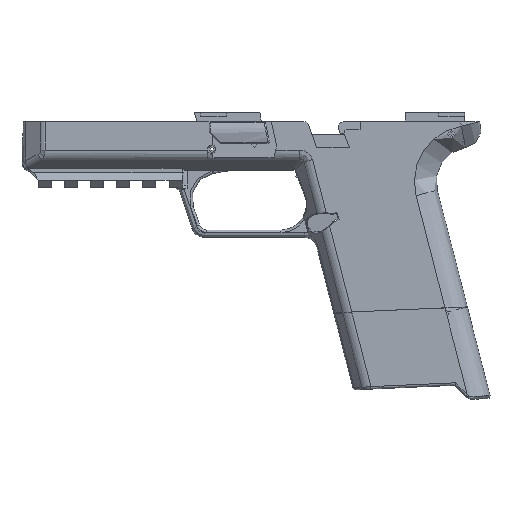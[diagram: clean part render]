
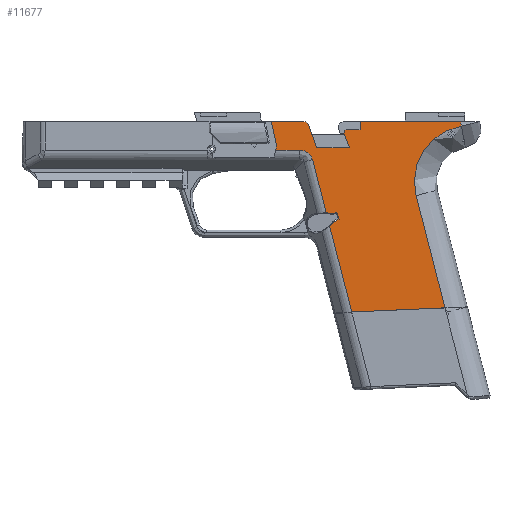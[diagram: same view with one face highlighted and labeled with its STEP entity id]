
A CAD part, left-side view. The second image highlights one B-rep face of the part: STEP entity #11677.
In plain terms, the highlighted face is planar.
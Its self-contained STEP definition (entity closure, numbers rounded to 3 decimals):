
#155=ELLIPSE('',#12633,10.693,7.);
#763=PLANE('',#12628);
#1239=FACE_OUTER_BOUND('',#1904,.T.);
#1904=EDGE_LOOP('',(#9328,#9329,#9330,#9331,#9332,#9333,#9334,#9335,#9336,
#9337,#9338,#9339,#9340,#9341,#9342,#9343,#9344,#9345,#9346,#9347,#9348,
#9349,#9350,#9351,#9352));
#2806=LINE('',#19325,#3937);
#2812=LINE('',#19335,#3943);
#2816=LINE('',#19343,#3947);
#2827=LINE('',#19402,#3958);
#2853=LINE('',#19467,#3984);
#2854=LINE('',#19469,#3985);
#2855=LINE('',#19471,#3986);
#2856=LINE('',#19477,#3987);
#2857=LINE('',#19479,#3988);
#2858=LINE('',#19481,#3989);
#2859=LINE('',#19485,#3990);
#2860=LINE('',#19487,#3991);
#2861=LINE('',#19489,#3992);
#2862=LINE('',#19493,#3993);
#2863=LINE('',#19495,#3994);
#2864=LINE('',#19497,#3995);
#2865=LINE('',#19499,#3996);
#2866=LINE('',#19502,#3997);
#3937=VECTOR('',#14691,10.);
#3943=VECTOR('',#14701,10.);
#3947=VECTOR('',#14709,10.);
#3958=VECTOR('',#14742,10.);
#3984=VECTOR('',#14802,10.);
#3985=VECTOR('',#14803,10.);
#3986=VECTOR('',#14804,10.);
#3987=VECTOR('',#14809,10.);
#3988=VECTOR('',#14810,10.);
#3989=VECTOR('',#14811,10.);
#3990=VECTOR('',#14814,10.);
#3991=VECTOR('',#14815,10.);
#3992=VECTOR('',#14816,10.);
#3993=VECTOR('',#14819,10.);
#3994=VECTOR('',#14820,10.);
#3995=VECTOR('',#14821,10.);
#3996=VECTOR('',#14822,10.);
#3997=VECTOR('',#14825,10.);
#4660=CIRCLE('',#12602,2.822);
#4661=CIRCLE('',#12606,2.822);
#4663=CIRCLE('',#12629,22.475);
#4664=CIRCLE('',#12630,7.5);
#4665=CIRCLE('',#12631,1.);
#4666=CIRCLE('',#12632,2.);
#5358=VERTEX_POINT('',#19322);
#5359=VERTEX_POINT('',#19324);
#5361=VERTEX_POINT('',#19333);
#5363=VERTEX_POINT('',#19342);
#5366=VERTEX_POINT('',#19356);
#5368=VERTEX_POINT('',#19363);
#5378=VERTEX_POINT('',#19400);
#5400=VERTEX_POINT('',#19466);
#5401=VERTEX_POINT('',#19468);
#5402=VERTEX_POINT('',#19470);
#5403=VERTEX_POINT('',#19472);
#5404=VERTEX_POINT('',#19474);
#5405=VERTEX_POINT('',#19476);
#5406=VERTEX_POINT('',#19478);
#5407=VERTEX_POINT('',#19480);
#5408=VERTEX_POINT('',#19482);
#5409=VERTEX_POINT('',#19484);
#5410=VERTEX_POINT('',#19486);
#5411=VERTEX_POINT('',#19488);
#5412=VERTEX_POINT('',#19490);
#5413=VERTEX_POINT('',#19492);
#5414=VERTEX_POINT('',#19494);
#5415=VERTEX_POINT('',#19496);
#5416=VERTEX_POINT('',#19498);
#5417=VERTEX_POINT('',#19500);
#6751=EDGE_CURVE('',#5359,#5358,#2806,.T.);
#6757=EDGE_CURVE('',#5358,#5361,#2812,.T.);
#6761=EDGE_CURVE('',#5363,#5359,#2816,.T.);
#6765=EDGE_CURVE('',#5361,#5366,#4660,.T.);
#6768=EDGE_CURVE('',#5368,#5363,#4661,.T.);
#6782=EDGE_CURVE('',#5366,#5378,#2827,.T.);
#6815=EDGE_CURVE('',#5400,#5378,#2853,.T.);
#6816=EDGE_CURVE('',#5401,#5400,#2854,.T.);
#6817=EDGE_CURVE('',#5402,#5401,#2855,.T.);
#6818=EDGE_CURVE('',#5403,#5402,#4663,.T.);
#6819=EDGE_CURVE('',#5404,#5403,#4664,.T.);
#6820=EDGE_CURVE('',#5404,#5405,#2856,.T.);
#6821=EDGE_CURVE('',#5405,#5406,#2857,.F.);
#6822=EDGE_CURVE('',#5406,#5407,#2858,.T.);
#6823=EDGE_CURVE('',#5408,#5407,#4665,.T.);
#6824=EDGE_CURVE('',#5408,#5409,#2859,.F.);
#6825=EDGE_CURVE('',#5409,#5410,#2860,.T.);
#6826=EDGE_CURVE('',#5410,#5411,#2861,.F.);
#6827=EDGE_CURVE('',#5412,#5411,#4666,.T.);
#6828=EDGE_CURVE('',#5412,#5413,#2862,.T.);
#6829=EDGE_CURVE('',#5413,#5414,#2863,.T.);
#6830=EDGE_CURVE('',#5414,#5415,#2864,.T.);
#6831=EDGE_CURVE('',#5416,#5415,#2865,.T.);
#6832=EDGE_CURVE('',#5417,#5416,#155,.T.);
#6833=EDGE_CURVE('',#5368,#5417,#2866,.T.);
#9328=ORIENTED_EDGE('',*,*,#6768,.T.);
#9329=ORIENTED_EDGE('',*,*,#6761,.T.);
#9330=ORIENTED_EDGE('',*,*,#6751,.T.);
#9331=ORIENTED_EDGE('',*,*,#6757,.T.);
#9332=ORIENTED_EDGE('',*,*,#6765,.T.);
#9333=ORIENTED_EDGE('',*,*,#6782,.T.);
#9334=ORIENTED_EDGE('',*,*,#6815,.F.);
#9335=ORIENTED_EDGE('',*,*,#6816,.F.);
#9336=ORIENTED_EDGE('',*,*,#6817,.F.);
#9337=ORIENTED_EDGE('',*,*,#6818,.F.);
#9338=ORIENTED_EDGE('',*,*,#6819,.F.);
#9339=ORIENTED_EDGE('',*,*,#6820,.T.);
#9340=ORIENTED_EDGE('',*,*,#6821,.T.);
#9341=ORIENTED_EDGE('',*,*,#6822,.T.);
#9342=ORIENTED_EDGE('',*,*,#6823,.F.);
#9343=ORIENTED_EDGE('',*,*,#6824,.T.);
#9344=ORIENTED_EDGE('',*,*,#6825,.T.);
#9345=ORIENTED_EDGE('',*,*,#6826,.T.);
#9346=ORIENTED_EDGE('',*,*,#6827,.F.);
#9347=ORIENTED_EDGE('',*,*,#6828,.T.);
#9348=ORIENTED_EDGE('',*,*,#6829,.T.);
#9349=ORIENTED_EDGE('',*,*,#6830,.T.);
#9350=ORIENTED_EDGE('',*,*,#6831,.F.);
#9351=ORIENTED_EDGE('',*,*,#6832,.F.);
#9352=ORIENTED_EDGE('',*,*,#6833,.F.);
#11677=ADVANCED_FACE('',(#1239),#763,.F.);
#12602=AXIS2_PLACEMENT_3D('',#19358,#14714,#14715);
#12606=AXIS2_PLACEMENT_3D('',#19364,#14722,#14723);
#12628=AXIS2_PLACEMENT_3D('',#19465,#14800,#14801);
#12629=AXIS2_PLACEMENT_3D('',#19473,#14805,#14806);
#12630=AXIS2_PLACEMENT_3D('',#19475,#14807,#14808);
#12631=AXIS2_PLACEMENT_3D('',#19483,#14812,#14813);
#12632=AXIS2_PLACEMENT_3D('',#19491,#14817,#14818);
#12633=AXIS2_PLACEMENT_3D('',#19501,#14823,#14824);
#14691=DIRECTION('',(0.,-0.323,0.947));
#14701=DIRECTION('',(0.,0.866,0.5));
#14709=DIRECTION('',(0.,-0.991,-0.133));
#14714=DIRECTION('center_axis',(-1.,0.,0.));
#14715=DIRECTION('ref_axis',(0.,-0.56,0.828));
#14722=DIRECTION('center_axis',(-1.,0.,0.));
#14723=DIRECTION('ref_axis',(0.,-0.504,-0.864));
#14742=DIRECTION('',(0.,0.828,0.56));
#14800=DIRECTION('center_axis',(-1.,0.,0.));
#14801=DIRECTION('ref_axis',(0.,1.,0.));
#14802=DIRECTION('',(0.,0.249,-0.969));
#14803=DIRECTION('',(0.,0.999,0.044));
#14804=DIRECTION('',(0.,-0.249,0.969));
#14805=DIRECTION('center_axis',(1.,0.,0.));
#14806=DIRECTION('ref_axis',(0.,0.,1.));
#14807=DIRECTION('center_axis',(1.,0.,0.));
#14808=DIRECTION('ref_axis',(0.,-0.97,-0.244));
#14809=DIRECTION('',(0.,1.,0.));
#14810=DIRECTION('',(0.,0.,-1.));
#14811=DIRECTION('',(0.,1.,0.));
#14812=DIRECTION('center_axis',(-1.,0.,0.));
#14813=DIRECTION('ref_axis',(0.,0.817,-0.576));
#14814=DIRECTION('',(0.,0.336,-0.942));
#14815=DIRECTION('',(0.,1.,0.));
#14816=DIRECTION('',(0.,-0.336,0.942));
#14817=DIRECTION('center_axis',(-1.,0.,0.));
#14818=DIRECTION('ref_axis',(0.,-0.576,-0.817));
#14819=DIRECTION('',(0.,1.,0.));
#14820=DIRECTION('',(0.,-0.21,0.978));
#14821=DIRECTION('',(0.,0.21,0.978));
#14822=DIRECTION('',(0.,1.,0.));
#14823=DIRECTION('center_axis',(1.,0.,0.));
#14824=DIRECTION('ref_axis',(0.,-0.714,-0.7));
#14825=DIRECTION('',(0.,0.249,-0.969));
#19322=CARTESIAN_POINT('',(22.175,-32.382,31.415));
#19324=CARTESIAN_POINT('',(22.175,-31.529,28.913));
#19325=CARTESIAN_POINT('',(22.175,-26.222,13.336));
#19333=CARTESIAN_POINT('',(22.175,-30.028,32.774));
#19335=CARTESIAN_POINT('',(22.175,-29.537,33.057));
#19342=CARTESIAN_POINT('',(22.175,-28.835,29.274));
#19343=CARTESIAN_POINT('',(22.175,-20.345,30.412));
#19356=CARTESIAN_POINT('',(22.175,-28.995,34.049));
#19358=CARTESIAN_POINT('Origin',(22.175,-27.413,31.712));
#19363=CARTESIAN_POINT('',(22.175,-27.244,28.895));
#19364=CARTESIAN_POINT('Origin',(22.175,-27.413,31.712));
#19400=CARTESIAN_POINT('',(22.175,-28.632,34.294));
#19402=CARTESIAN_POINT('',(22.175,-29.16,33.937));
#19465=CARTESIAN_POINT('Origin',(22.175,-7.921,2.186));
#19466=CARTESIAN_POINT('',(22.175,-37.447,68.587));
#19467=CARTESIAN_POINT('',(22.175,-26.659,26.619));
#19468=CARTESIAN_POINT('',(22.175,-74.722,66.935));
#19469=CARTESIAN_POINT('',(22.175,-40.785,68.439));
#19470=CARTESIAN_POINT('',(22.175,-63.184,22.049));
#19471=CARTESIAN_POINT('',(22.175,-75.103,68.418));
#19472=CARTESIAN_POINT('',(22.175,-81.332,-5.728));
#19473=CARTESIAN_POINT('Origin',(22.175,-84.951,16.453));
#19474=CARTESIAN_POINT('',(22.175,-81.106,-7.556));
#19475=CARTESIAN_POINT('Origin',(22.175,-88.606,-7.556));
#19476=CARTESIAN_POINT('',(22.175,-40.774,-7.556));
#19477=CARTESIAN_POINT('',(22.175,-84.951,-7.556));
#19478=CARTESIAN_POINT('',(22.175,-40.774,-4.331));
#19479=CARTESIAN_POINT('',(22.175,-40.774,-2.685));
#19480=CARTESIAN_POINT('',(22.175,-35.316,-4.331));
#19481=CARTESIAN_POINT('',(22.175,-20.598,-4.331));
#19482=CARTESIAN_POINT('',(22.175,-34.374,-2.995));
#19483=CARTESIAN_POINT('Origin',(22.175,-35.316,-3.331));
#19484=CARTESIAN_POINT('',(22.175,-36.514,3.));
#19485=CARTESIAN_POINT('',(22.175,-32.976,-6.913));
#19486=CARTESIAN_POINT('',(22.175,-23.407,3.));
#19487=CARTESIAN_POINT('',(22.175,-23.764,3.));
#19488=CARTESIAN_POINT('',(22.175,-20.114,-6.228));
#19489=CARTESIAN_POINT('',(22.175,-21.552,-2.199));
#19490=CARTESIAN_POINT('',(22.175,-18.23,-7.556));
#19491=CARTESIAN_POINT('Origin',(22.175,-18.23,-5.556));
#19492=CARTESIAN_POINT('',(22.175,-5.3,-7.556));
#19493=CARTESIAN_POINT('',(22.175,-86.951,-7.556));
#19494=CARTESIAN_POINT('',(22.175,-7.389,2.186));
#19495=CARTESIAN_POINT('',(22.175,-6.356,-2.63));
#19496=CARTESIAN_POINT('',(22.175,-7.025,3.884));
#19497=CARTESIAN_POINT('',(22.175,-7.4,2.132));
#19498=CARTESIAN_POINT('',(22.175,-16.536,3.884));
#19499=CARTESIAN_POINT('',(22.175,33.814,3.884));
#19500=CARTESIAN_POINT('',(22.175,-21.783,7.651));
#19501=CARTESIAN_POINT('Origin',(22.175,-12.907,12.884));
#19502=CARTESIAN_POINT('',(22.175,-26.659,26.619));
